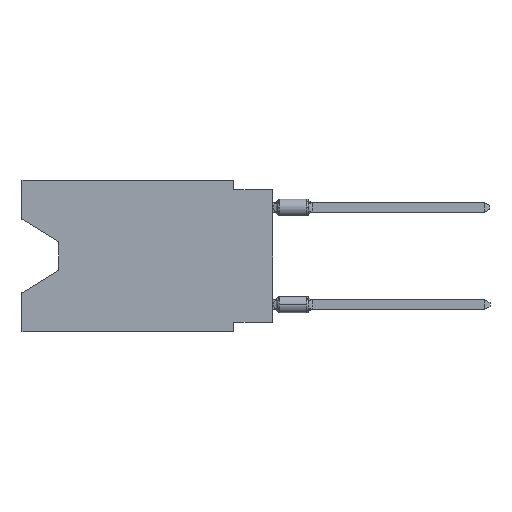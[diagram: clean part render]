
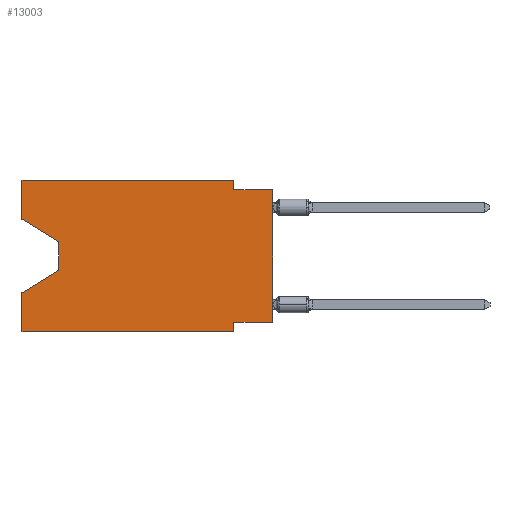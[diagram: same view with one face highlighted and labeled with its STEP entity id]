
A CAD part, left-side view. The second image highlights one B-rep face of the part: STEP entity #13003.
In plain terms, the highlighted planar face has unit normal (-1, 0, 0).
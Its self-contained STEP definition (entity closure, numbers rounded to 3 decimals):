
#14 = ORIENTED_EDGE ( 'NONE', *, *, #4468, .T. ) ;
#538 = LINE ( 'NONE', #7588, #16261 ) ;
#555 = CARTESIAN_POINT ( 'NONE',  ( 0., 16.383, -7.36 ) ) ;
#774 = CARTESIAN_POINT ( 'NONE',  ( 0., 13.97, -4.013 ) ) ;
#1170 = VERTEX_POINT ( 'NONE', #12787 ) ;
#1230 = EDGE_CURVE ( 'NONE', #1170, #11009, #8356, .T. ) ;
#1377 = ORIENTED_EDGE ( 'NONE', *, *, #9864, .F. ) ;
#1409 = CARTESIAN_POINT ( 'NONE',  ( 0., 0., -9.271 ) ) ;
#1751 = VERTEX_POINT ( 'NONE', #2890 ) ;
#2201 = DIRECTION ( 'NONE',  ( 0., 0., -1. ) ) ;
#2299 = DIRECTION ( 'NONE',  ( 1., 0., 0. ) ) ;
#2489 = ORIENTED_EDGE ( 'NONE', *, *, #12912, .F. ) ;
#2738 = VERTEX_POINT ( 'NONE', #5152 ) ;
#2890 = CARTESIAN_POINT ( 'NONE',  ( 0., 13.97, -5.893 ) ) ;
#3186 = ORIENTED_EDGE ( 'NONE', *, *, #17240, .F. ) ;
#3834 = EDGE_CURVE ( 'NONE', #11969, #2738, #13273, .T. ) ;
#4327 = LINE ( 'NONE', #8740, #7530 ) ;
#4468 = EDGE_CURVE ( 'NONE', #14431, #6331, #15219, .T. ) ;
#4558 = CARTESIAN_POINT ( 'NONE',  ( 0., 0., -9.271 ) ) ;
#4807 = CARTESIAN_POINT ( 'NONE',  ( 0., 16.383, 0. ) ) ;
#5152 = CARTESIAN_POINT ( 'NONE',  ( 0., 16.383, 0. ) ) ;
#5221 = LINE ( 'NONE', #10960, #7563 ) ;
#5231 = DIRECTION ( 'NONE',  ( 0., -1., 0. ) ) ;
#5283 = ORIENTED_EDGE ( 'NONE', *, *, #10088, .T. ) ;
#5417 = VERTEX_POINT ( 'NONE', #1409 ) ;
#5544 = DIRECTION ( 'NONE',  ( 0., 0., -1. ) ) ;
#5653 = VERTEX_POINT ( 'NONE', #6187 ) ;
#5932 = CARTESIAN_POINT ( 'NONE',  ( 0., 13.97, -4.013 ) ) ;
#6170 = VECTOR ( 'NONE', #10295, 1000. ) ;
#6187 = CARTESIAN_POINT ( 'NONE',  ( 0., 0., -0.635 ) ) ;
#6230 = LINE ( 'NONE', #11977, #9359 ) ;
#6331 = VERTEX_POINT ( 'NONE', #15750 ) ;
#6608 = CARTESIAN_POINT ( 'NONE',  ( 0., 16.383, 0. ) ) ;
#7050 = VECTOR ( 'NONE', #5544, 1000. ) ;
#7160 = DIRECTION ( 'NONE',  ( 0., -1., 0. ) ) ;
#7363 = VERTEX_POINT ( 'NONE', #15475 ) ;
#7530 = VECTOR ( 'NONE', #7160, 1000. ) ;
#7563 = VECTOR ( 'NONE', #16698, 1000. ) ;
#7588 = CARTESIAN_POINT ( 'NONE',  ( 0., 0., -0.635 ) ) ;
#7776 = VECTOR ( 'NONE', #10264, 1000. ) ;
#8167 = DIRECTION ( 'NONE',  ( 0., 0., -1. ) ) ;
#8308 = CARTESIAN_POINT ( 'NONE',  ( 0., 16.383, -2.546 ) ) ;
#8356 = LINE ( 'NONE', #14111, #8906 ) ;
#8433 = VERTEX_POINT ( 'NONE', #555 ) ;
#8740 = CARTESIAN_POINT ( 'NONE',  ( 0., 16.383, 0. ) ) ;
#8906 = VECTOR ( 'NONE', #8167, 1000. ) ;
#9359 = VECTOR ( 'NONE', #17704, 1000. ) ;
#9497 = ORIENTED_EDGE ( 'NONE', *, *, #11630, .T. ) ;
#9547 = EDGE_CURVE ( 'NONE', #5417, #5653, #16190, .T. ) ;
#9599 = VECTOR ( 'NONE', #14066, 1000. ) ;
#9864 = EDGE_CURVE ( 'NONE', #11009, #5653, #538, .T. ) ;
#9923 = VECTOR ( 'NONE', #11675, 1000. ) ;
#9974 = CARTESIAN_POINT ( 'NONE',  ( 0., 16.383, -2.546 ) ) ;
#10088 = EDGE_CURVE ( 'NONE', #1751, #8433, #5221, .T. ) ;
#10139 = ORIENTED_EDGE ( 'NONE', *, *, #1230, .F. ) ;
#10264 = DIRECTION ( 'NONE',  ( 0., 0., 1. ) ) ;
#10295 = DIRECTION ( 'NONE',  ( 0., 1., 0. ) ) ;
#10688 = VECTOR ( 'NONE', #5231, 1000. ) ;
#10715 = VECTOR ( 'NONE', #16374, 1000. ) ;
#10851 = PLANE ( 'NONE',  #16681 ) ;
#10960 = CARTESIAN_POINT ( 'NONE',  ( 0., 13.97, -5.893 ) ) ;
#11009 = VERTEX_POINT ( 'NONE', #13347 ) ;
#11094 = LINE ( 'NONE', #16828, #7050 ) ;
#11193 = ORIENTED_EDGE ( 'NONE', *, *, #11839, .T. ) ;
#11630 = EDGE_CURVE ( 'NONE', #11969, #16107, #15741, .T. ) ;
#11675 = DIRECTION ( 'NONE',  ( 0., 0., -1. ) ) ;
#11839 = EDGE_CURVE ( 'NONE', #16107, #1751, #17037, .T. ) ;
#11868 = EDGE_CURVE ( 'NONE', #2738, #1170, #4327, .T. ) ;
#11969 = VERTEX_POINT ( 'NONE', #9974 ) ;
#11977 = CARTESIAN_POINT ( 'NONE',  ( 0., 16.383, 0. ) ) ;
#12443 = FACE_OUTER_BOUND ( 'NONE', #14748, .T. ) ;
#12787 = CARTESIAN_POINT ( 'NONE',  ( 0., 2.54, 0. ) ) ;
#12912 = EDGE_CURVE ( 'NONE', #5417, #7363, #17364, .T. ) ;
#13003 = ADVANCED_FACE ( 'NONE', ( #12443 ), #10851, .F. ) ;
#13273 = LINE ( 'NONE', #4807, #10715 ) ;
#13323 = DIRECTION ( 'NONE',  ( 0., -1., 0. ) ) ;
#13347 = CARTESIAN_POINT ( 'NONE',  ( 0., 2.54, -0.635 ) ) ;
#13990 = CARTESIAN_POINT ( 'NONE',  ( 0., 16.383, -9.906 ) ) ;
#14066 = DIRECTION ( 'NONE',  ( 0., -0.855, -0.519 ) ) ;
#14111 = CARTESIAN_POINT ( 'NONE',  ( 0., 2.54, 0. ) ) ;
#14431 = VERTEX_POINT ( 'NONE', #14801 ) ;
#14706 = ORIENTED_EDGE ( 'NONE', *, *, #3834, .F. ) ;
#14748 = EDGE_LOOP ( 'NONE', ( #9497, #11193, #5283, #3186, #14, #15969, #2489, #18305, #1377, #10139, #16591, #14706 ) ) ;
#14801 = CARTESIAN_POINT ( 'NONE',  ( 0., 16.383, -9.906 ) ) ;
#15219 = LINE ( 'NONE', #13990, #10688 ) ;
#15257 = EDGE_CURVE ( 'NONE', #7363, #6331, #11094, .T. ) ;
#15475 = CARTESIAN_POINT ( 'NONE',  ( 0., 2.54, -9.271 ) ) ;
#15741 = LINE ( 'NONE', #8308, #9599 ) ;
#15750 = CARTESIAN_POINT ( 'NONE',  ( 0., 2.54, -9.906 ) ) ;
#15969 = ORIENTED_EDGE ( 'NONE', *, *, #15257, .F. ) ;
#16107 = VERTEX_POINT ( 'NONE', #774 ) ;
#16190 = LINE ( 'NONE', #17413, #7776 ) ;
#16261 = VECTOR ( 'NONE', #13323, 1000. ) ;
#16374 = DIRECTION ( 'NONE',  ( 0., 0., 1. ) ) ;
#16591 = ORIENTED_EDGE ( 'NONE', *, *, #11868, .F. ) ;
#16681 = AXIS2_PLACEMENT_3D ( 'NONE', #6608, #2299, #2201 ) ;
#16698 = DIRECTION ( 'NONE',  ( 0., 0.855, -0.519 ) ) ;
#16828 = CARTESIAN_POINT ( 'NONE',  ( 0., 2.54, -9.906 ) ) ;
#17037 = LINE ( 'NONE', #5932, #9923 ) ;
#17240 = EDGE_CURVE ( 'NONE', #14431, #8433, #6230, .T. ) ;
#17364 = LINE ( 'NONE', #4558, #6170 ) ;
#17413 = CARTESIAN_POINT ( 'NONE',  ( 0., 0., 0. ) ) ;
#17704 = DIRECTION ( 'NONE',  ( 0., 0., 1. ) ) ;
#18305 = ORIENTED_EDGE ( 'NONE', *, *, #9547, .T. ) ;
